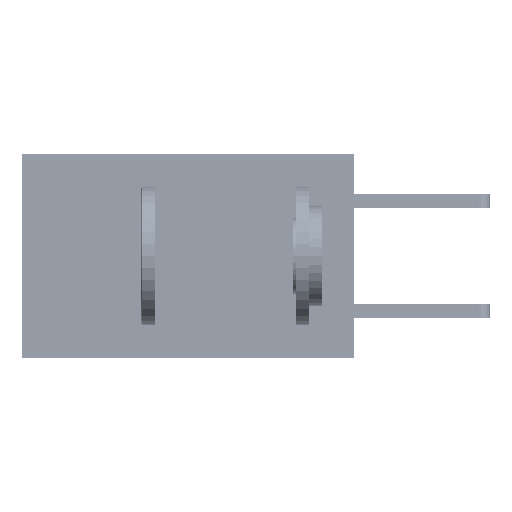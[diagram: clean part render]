
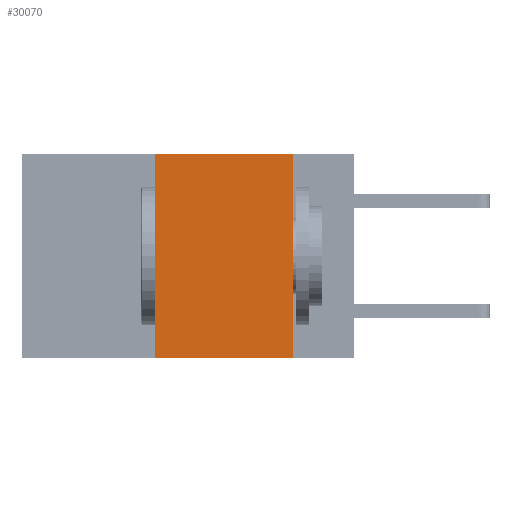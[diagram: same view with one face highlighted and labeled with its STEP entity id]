
A CAD part, left-side view. The second image highlights one B-rep face of the part: STEP entity #30070.
In plain terms, the highlighted planar face has unit normal (-1, 0, 0).
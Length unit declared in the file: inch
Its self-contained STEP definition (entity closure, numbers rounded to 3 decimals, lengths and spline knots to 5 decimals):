
#2284 = VERTEX_POINT ( 'NONE', #4622 ) ;
#3987 = CARTESIAN_POINT ( 'NONE',  ( 0., 0.11, 0. ) ) ;
#4622 = CARTESIAN_POINT ( 'NONE',  ( 0., 0.11, -0.37 ) ) ;
#6606 = EDGE_CURVE ( 'NONE', #26447, #26015, #44576, .T. ) ;
#8391 = DIRECTION ( 'NONE',  ( 0., -1., 0. ) ) ;
#10289 = CARTESIAN_POINT ( 'NONE',  ( 0., 0.36, 0. ) ) ;
#11834 = VECTOR ( 'NONE', #30936, 39.37008 ) ;
#12172 = ORIENTED_EDGE ( 'NONE', *, *, #31578, .T. ) ;
#12731 = CARTESIAN_POINT ( 'NONE',  ( 0., 0.6, 0. ) ) ;
#15392 = CARTESIAN_POINT ( 'NONE',  ( 0., 0.6, -0.37 ) ) ;
#16462 = LINE ( 'NONE', #12731, #11834 ) ;
#16479 = AXIS2_PLACEMENT_3D ( 'NONE', #16809, #27531, #28222 ) ;
#16809 = CARTESIAN_POINT ( 'NONE',  ( 0., 0.6, 0. ) ) ;
#17272 = FACE_OUTER_BOUND ( 'NONE', #36943, .T. ) ;
#19254 = ORIENTED_EDGE ( 'NONE', *, *, #20180, .F. ) ;
#20180 = EDGE_CURVE ( 'NONE', #26015, #34227, #16462, .T. ) ;
#21247 = DIRECTION ( 'NONE',  ( 0., 0., -1. ) ) ;
#26015 = VERTEX_POINT ( 'NONE', #10289 ) ;
#26447 = VERTEX_POINT ( 'NONE', #43841 ) ;
#27531 = DIRECTION ( 'NONE',  ( 1., 0., 0. ) ) ;
#28222 = DIRECTION ( 'NONE',  ( 0., 0., -1. ) ) ;
#29968 = VECTOR ( 'NONE', #21247, 39.37008 ) ;
#30070 = ADVANCED_FACE ( 'NONE', ( #17272 ), #31955, .F. ) ;
#30936 = DIRECTION ( 'NONE',  ( 0., -1., 0. ) ) ;
#31578 = EDGE_CURVE ( 'NONE', #26447, #2284, #32892, .T. ) ;
#31955 = PLANE ( 'NONE',  #16479 ) ;
#32892 = LINE ( 'NONE', #15392, #34358 ) ;
#34164 = EDGE_CURVE ( 'NONE', #34227, #2284, #43147, .T. ) ;
#34227 = VERTEX_POINT ( 'NONE', #3987 ) ;
#34358 = VECTOR ( 'NONE', #8391, 39.37008 ) ;
#36943 = EDGE_LOOP ( 'NONE', ( #43328, #19254, #44841, #12172 ) ) ;
#37819 = DIRECTION ( 'NONE',  ( 0., 0., 1. ) ) ;
#40410 = VECTOR ( 'NONE', #37819, 39.37008 ) ;
#42231 = CARTESIAN_POINT ( 'NONE',  ( 0., 0.11, 0. ) ) ;
#43147 = LINE ( 'NONE', #42231, #29968 ) ;
#43328 = ORIENTED_EDGE ( 'NONE', *, *, #34164, .F. ) ;
#43841 = CARTESIAN_POINT ( 'NONE',  ( 0., 0.36, -0.37 ) ) ;
#44576 = LINE ( 'NONE', #45034, #40410 ) ;
#44841 = ORIENTED_EDGE ( 'NONE', *, *, #6606, .F. ) ;
#45034 = CARTESIAN_POINT ( 'NONE',  ( 0., 0.36, 0. ) ) ;
